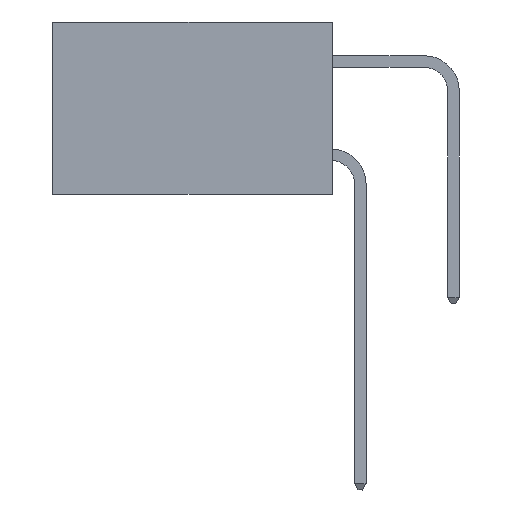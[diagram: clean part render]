
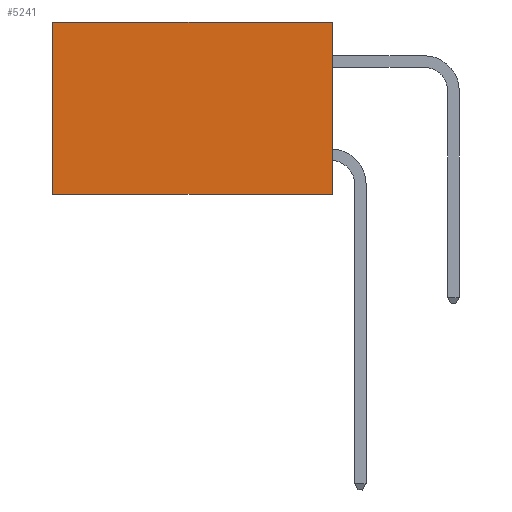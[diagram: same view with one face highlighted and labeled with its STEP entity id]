
A CAD part, left-side view. The second image highlights one B-rep face of the part: STEP entity #5241.
In plain terms, the highlighted planar face has unit normal (-1, 0, 0).
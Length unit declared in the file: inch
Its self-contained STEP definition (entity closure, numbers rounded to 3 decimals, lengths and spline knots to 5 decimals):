
#263 = VERTEX_POINT ( 'NONE', #16095 ) ;
#1389 = DIRECTION ( 'NONE',  ( 0., 0., -1. ) ) ;
#1576 = ORIENTED_EDGE ( 'NONE', *, *, #20578, .T. ) ;
#3562 = VECTOR ( 'NONE', #18522, 39.37008 ) ;
#4333 = LINE ( 'NONE', #11206, #3562 ) ;
#4616 = CARTESIAN_POINT ( 'NONE',  ( 0.298, 0., 0. ) ) ;
#5241 = ADVANCED_FACE ( 'NONE', ( #17469 ), #28273, .F. ) ;
#6482 = DIRECTION ( 'NONE',  ( 0., 0., -1. ) ) ;
#7008 = CARTESIAN_POINT ( 'NONE',  ( 0.298, 0., 0. ) ) ;
#7079 = DIRECTION ( 'NONE',  ( 0., 1., 0. ) ) ;
#7667 = CARTESIAN_POINT ( 'NONE',  ( 0.298, 0., -0.37 ) ) ;
#8764 = EDGE_LOOP ( 'NONE', ( #1576, #28543, #30877, #22621 ) ) ;
#9370 = VECTOR ( 'NONE', #10116, 39.37008 ) ;
#10116 = DIRECTION ( 'NONE',  ( 0., 1., 0. ) ) ;
#11206 = CARTESIAN_POINT ( 'NONE',  ( 0.298, 0.6, 0. ) ) ;
#11285 = CARTESIAN_POINT ( 'NONE',  ( 0.298, 0.6, 0. ) ) ;
#11608 = VECTOR ( 'NONE', #7079, 39.37008 ) ;
#13707 = CARTESIAN_POINT ( 'NONE',  ( 0.298, 0., 0. ) ) ;
#14905 = VECTOR ( 'NONE', #1389, 39.37008 ) ;
#16095 = CARTESIAN_POINT ( 'NONE',  ( 0.298, 0.6, -0.37 ) ) ;
#17469 = FACE_OUTER_BOUND ( 'NONE', #8764, .T. ) ;
#18522 = DIRECTION ( 'NONE',  ( 0., 0., -1. ) ) ;
#19368 = LINE ( 'NONE', #7667, #9370 ) ;
#20080 = EDGE_CURVE ( 'NONE', #21544, #21378, #24559, .T. ) ;
#20578 = EDGE_CURVE ( 'NONE', #21378, #263, #4333, .T. ) ;
#21075 = AXIS2_PLACEMENT_3D ( 'NONE', #13707, #21076, #6482 ) ;
#21076 = DIRECTION ( 'NONE',  ( 1., 0., 0. ) ) ;
#21378 = VERTEX_POINT ( 'NONE', #11285 ) ;
#21544 = VERTEX_POINT ( 'NONE', #7008 ) ;
#22621 = ORIENTED_EDGE ( 'NONE', *, *, #20080, .T. ) ;
#23118 = EDGE_CURVE ( 'NONE', #28943, #263, #19368, .T. ) ;
#24559 = LINE ( 'NONE', #4616, #11608 ) ;
#24959 = CARTESIAN_POINT ( 'NONE',  ( 0.298, 0., -0.37 ) ) ;
#27859 = LINE ( 'NONE', #30497, #14905 ) ;
#28273 = PLANE ( 'NONE',  #21075 ) ;
#28485 = EDGE_CURVE ( 'NONE', #21544, #28943, #27859, .T. ) ;
#28543 = ORIENTED_EDGE ( 'NONE', *, *, #23118, .F. ) ;
#28943 = VERTEX_POINT ( 'NONE', #24959 ) ;
#30497 = CARTESIAN_POINT ( 'NONE',  ( 0.298, 0., 0. ) ) ;
#30877 = ORIENTED_EDGE ( 'NONE', *, *, #28485, .F. ) ;
